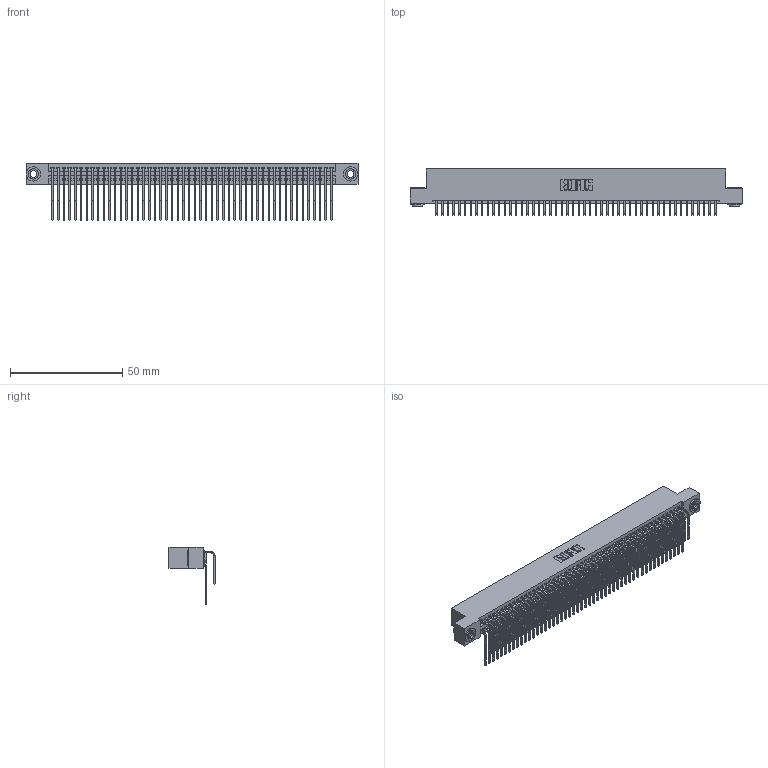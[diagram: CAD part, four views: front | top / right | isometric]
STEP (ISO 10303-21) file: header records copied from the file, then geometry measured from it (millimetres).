
FILE_DESCRIPTION (( 'STEP AP203' ), '1' );
FILE_NAME ('345-100-559-203.STEP', '2018-10-05T17:22:33', ( '' ), ( '' ), 'SwSTEP 2.0', 'SolidWorks 2016', '' );
FILE_SCHEMA (( 'CONFIG_CONTROL_DESIGN' ));
Length unit declared in the file: inch
Products named in the file (5): 345-292-001_558 559 Tail - 1; 345-250-002_345-250-002-102; 345-292-001_559 Tail - 2; 345 Part_Flush Mounting Lugs - 0.156 Dia-TH; 345-100-559-203
Assembly tree (103 placements, depth 2):
  345-100-559-203
    345 Part_Flush Mounting Lugs - 0.156 Dia-TH
    345-292-001_558 559 Tail - 1  x50
    345-292-001_559 Tail - 2  x50
    345-250-002_345-250-002-102  x2
Bounding box: 148.21 x 20.56 x 25.53 mm (x, y, z)
Volume: 15067.7 mm3; surface area: 25345.1 mm2
Topology: 103 solids, 103 shells, 5364 faces, 15917 edges, 10474 vertices
Faces by surface type: plane 3590, cylinder 1766, cone 8
Entity records: 40456 total; most frequent: CARTESIAN_POINT 6794, ORIENTED_EDGE 6670, DIRECTION 5985, EDGE_CURVE 3335, LINE 2939, VECTOR 2939, VERTEX_POINT 2218, AXIS2_PLACEMENT_3D 1523
